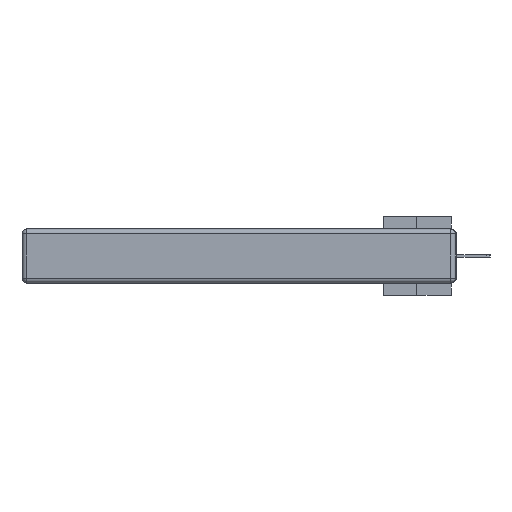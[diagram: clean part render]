
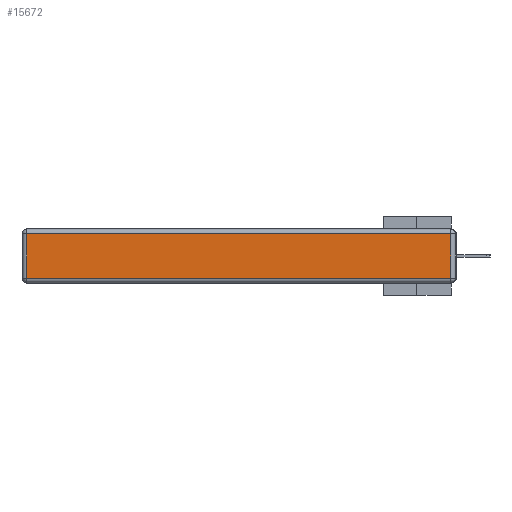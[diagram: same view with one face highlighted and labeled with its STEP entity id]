
A CAD part, left-side view. The second image highlights one B-rep face of the part: STEP entity #15672.
In plain terms, the highlighted planar face has unit normal (-1, 0, 0).
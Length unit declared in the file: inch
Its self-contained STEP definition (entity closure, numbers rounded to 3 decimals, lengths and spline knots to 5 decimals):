
#1262 = LINE ( 'NONE', #22059, #17666 ) ;
#2292 = ORIENTED_EDGE ( 'NONE', *, *, #36033, .T. ) ;
#2619 = CARTESIAN_POINT ( 'NONE',  ( 0., 2.72, -0.313 ) ) ;
#2917 = CARTESIAN_POINT ( 'NONE',  ( 0., 0., -0.343 ) ) ;
#3635 = CARTESIAN_POINT ( 'NONE',  ( 0., 2.75, -0.03 ) ) ;
#4270 = DIRECTION ( 'NONE',  ( 0., 0., -1. ) ) ;
#5330 = VERTEX_POINT ( 'NONE', #2619 ) ;
#6118 = DIRECTION ( 'NONE',  ( -1., 0., 0. ) ) ;
#6423 = CARTESIAN_POINT ( 'NONE',  ( 0., 2.72, -0.03 ) ) ;
#7155 = CARTESIAN_POINT ( 'NONE',  ( 0., 0.03, -0.313 ) ) ;
#8418 = LINE ( 'NONE', #37564, #14635 ) ;
#9744 = EDGE_CURVE ( 'NONE', #5330, #17872, #12331, .T. ) ;
#11069 = VERTEX_POINT ( 'NONE', #16158 ) ;
#12032 = EDGE_LOOP ( 'NONE', ( #38895, #24829, #33789, #2292 ) ) ;
#12331 = LINE ( 'NONE', #23054, #35450 ) ;
#14635 = VECTOR ( 'NONE', #4270, 39.37008 ) ;
#15672 = ADVANCED_FACE ( 'NONE', ( #26302 ), #21274, .T. ) ;
#16158 = CARTESIAN_POINT ( 'NONE',  ( 0., 0.03, -0.03 ) ) ;
#17666 = VECTOR ( 'NONE', #34179, 39.37008 ) ;
#17830 = EDGE_CURVE ( 'NONE', #17872, #11069, #1262, .T. ) ;
#17872 = VERTEX_POINT ( 'NONE', #7155 ) ;
#21274 = PLANE ( 'NONE',  #26252 ) ;
#21277 = VERTEX_POINT ( 'NONE', #6423 ) ;
#21976 = DIRECTION ( 'NONE',  ( 0., 1., 0. ) ) ;
#22059 = CARTESIAN_POINT ( 'NONE',  ( 0., 0.03, -0.343 ) ) ;
#23054 = CARTESIAN_POINT ( 'NONE',  ( 0., 0., -0.313 ) ) ;
#23117 = LINE ( 'NONE', #3635, #38155 ) ;
#24829 = ORIENTED_EDGE ( 'NONE', *, *, #17830, .T. ) ;
#26252 = AXIS2_PLACEMENT_3D ( 'NONE', #2917, #6118, #27349 ) ;
#26302 = FACE_OUTER_BOUND ( 'NONE', #12032, .T. ) ;
#27349 = DIRECTION ( 'NONE',  ( 0., 0., 1. ) ) ;
#29981 = EDGE_CURVE ( 'NONE', #11069, #21277, #23117, .T. ) ;
#32158 = DIRECTION ( 'NONE',  ( 0., -1., 0. ) ) ;
#33789 = ORIENTED_EDGE ( 'NONE', *, *, #29981, .T. ) ;
#34179 = DIRECTION ( 'NONE',  ( 0., 0., 1. ) ) ;
#35450 = VECTOR ( 'NONE', #32158, 39.37008 ) ;
#36033 = EDGE_CURVE ( 'NONE', #21277, #5330, #8418, .T. ) ;
#37564 = CARTESIAN_POINT ( 'NONE',  ( 0., 2.72, -0.343 ) ) ;
#38155 = VECTOR ( 'NONE', #21976, 39.37008 ) ;
#38895 = ORIENTED_EDGE ( 'NONE', *, *, #9744, .T. ) ;
